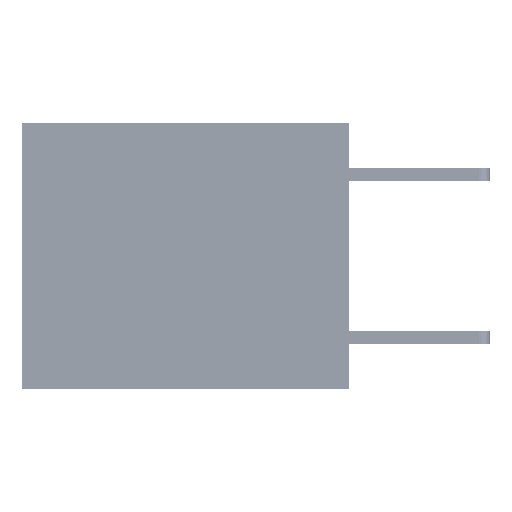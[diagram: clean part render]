
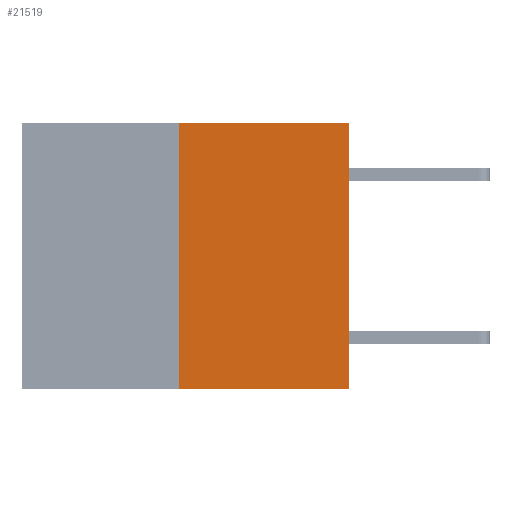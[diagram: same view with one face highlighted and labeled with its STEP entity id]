
A CAD part, left-side view. The second image highlights one B-rep face of the part: STEP entity #21519.
In plain terms, the highlighted planar face has unit normal (-1, 0, 0).
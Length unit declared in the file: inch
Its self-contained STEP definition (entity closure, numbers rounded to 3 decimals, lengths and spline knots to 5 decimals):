
#527 = VERTEX_POINT ( 'NONE', #17461 ) ;
#1295 = AXIS2_PLACEMENT_3D ( 'NONE', #35137, #11843, #18328 ) ;
#2316 = ORIENTED_EDGE ( 'NONE', *, *, #25079, .F. ) ;
#3824 = VERTEX_POINT ( 'NONE', #18737 ) ;
#6577 = CARTESIAN_POINT ( 'NONE',  ( 0., 0.6, -0.49 ) ) ;
#7894 = VECTOR ( 'NONE', #13423, 39.37008 ) ;
#8678 = CARTESIAN_POINT ( 'NONE',  ( 0., 0.312, -0.49 ) ) ;
#9513 = DIRECTION ( 'NONE',  ( 0., -1., 0. ) ) ;
#10144 = EDGE_CURVE ( 'NONE', #23562, #24830, #19525, .T. ) ;
#10453 = VECTOR ( 'NONE', #9513, 39.37008 ) ;
#11735 = CARTESIAN_POINT ( 'NONE',  ( 0., 0.6, 0. ) ) ;
#11843 = DIRECTION ( 'NONE',  ( 1., 0., 0. ) ) ;
#11849 = DIRECTION ( 'NONE',  ( 0., 0., 1. ) ) ;
#13423 = DIRECTION ( 'NONE',  ( 0., 0., 1. ) ) ;
#16229 = CARTESIAN_POINT ( 'NONE',  ( 0., 0.312, -0.49 ) ) ;
#16961 = LINE ( 'NONE', #18151, #7894 ) ;
#17461 = CARTESIAN_POINT ( 'NONE',  ( 0., 0., 0. ) ) ;
#17873 = ORIENTED_EDGE ( 'NONE', *, *, #33949, .F. ) ;
#18151 = CARTESIAN_POINT ( 'NONE',  ( 0., 0., 0. ) ) ;
#18328 = DIRECTION ( 'NONE',  ( 0., 0., -1. ) ) ;
#18737 = CARTESIAN_POINT ( 'NONE',  ( 0., 0.312, 0. ) ) ;
#19335 = LINE ( 'NONE', #8678, #20268 ) ;
#19525 = LINE ( 'NONE', #6577, #10453 ) ;
#20268 = VECTOR ( 'NONE', #11849, 39.37008 ) ;
#21519 = ADVANCED_FACE ( 'NONE', ( #31667 ), #37441, .F. ) ;
#22559 = ORIENTED_EDGE ( 'NONE', *, *, #26713, .T. ) ;
#22833 = LINE ( 'NONE', #11735, #35275 ) ;
#23562 = VERTEX_POINT ( 'NONE', #16229 ) ;
#24830 = VERTEX_POINT ( 'NONE', #27913 ) ;
#25079 = EDGE_CURVE ( 'NONE', #23562, #3824, #19335, .T. ) ;
#25769 = EDGE_LOOP ( 'NONE', ( #2316, #32122, #22559, #17873 ) ) ;
#26713 = EDGE_CURVE ( 'NONE', #24830, #527, #16961, .T. ) ;
#27913 = CARTESIAN_POINT ( 'NONE',  ( 0., 0., -0.49 ) ) ;
#29383 = DIRECTION ( 'NONE',  ( 0., -1., 0. ) ) ;
#31667 = FACE_OUTER_BOUND ( 'NONE', #25769, .T. ) ;
#32122 = ORIENTED_EDGE ( 'NONE', *, *, #10144, .T. ) ;
#33949 = EDGE_CURVE ( 'NONE', #3824, #527, #22833, .T. ) ;
#35137 = CARTESIAN_POINT ( 'NONE',  ( 0., 0.6, 0. ) ) ;
#35275 = VECTOR ( 'NONE', #29383, 39.37008 ) ;
#37441 = PLANE ( 'NONE',  #1295 ) ;
